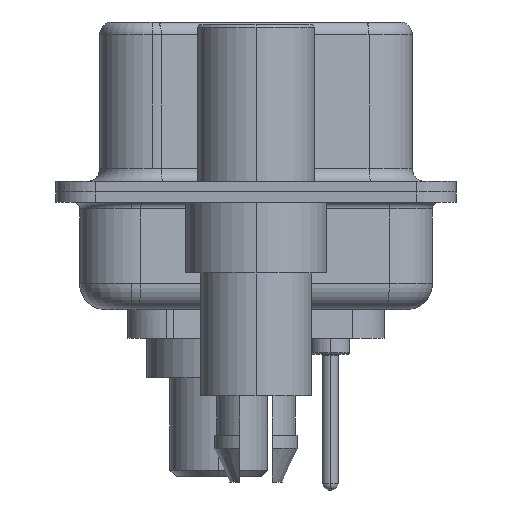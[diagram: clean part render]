
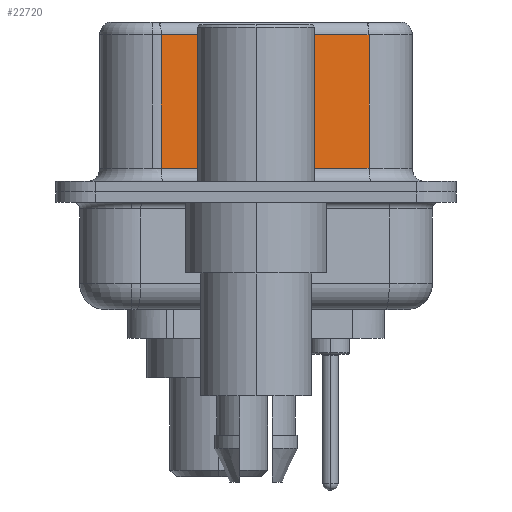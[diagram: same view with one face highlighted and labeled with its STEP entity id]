
A CAD part, left-side view. The second image highlights one B-rep face of the part: STEP entity #22720.
In plain terms, the highlighted planar face has unit normal (-0.985, -0.174, 0).
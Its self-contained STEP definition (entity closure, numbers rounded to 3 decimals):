
#587 = ORIENTED_EDGE ( 'NONE', *, *, #14747, .T. ) ;
#1280 = LINE ( 'NONE', #17066, #16430 ) ;
#2377 = EDGE_CURVE ( 'NONE', #8021, #12807, #23471, .T. ) ;
#3465 = DIRECTION ( 'NONE',  ( -0.174, 0.985, 0. ) ) ;
#3776 = DIRECTION ( 'NONE',  ( -0.174, 0.985, 0. ) ) ;
#4102 = CARTESIAN_POINT ( 'NONE',  ( 5.132, -4.322, 0.9 ) ) ;
#4895 = VERTEX_POINT ( 'NONE', #10823 ) ;
#5987 = DIRECTION ( 'NONE',  ( 0.174, -0.985, 0. ) ) ;
#6564 = ORIENTED_EDGE ( 'NONE', *, *, #2377, .F. ) ;
#7242 = AXIS2_PLACEMENT_3D ( 'NONE', #20576, #14840, #3465 ) ;
#7316 = LINE ( 'NONE', #14742, #21986 ) ;
#8021 = VERTEX_POINT ( 'NONE', #11078 ) ;
#8218 = VECTOR ( 'NONE', #22270, 1000. ) ;
#8408 = CARTESIAN_POINT ( 'NONE',  ( 5.132, -4.322, 6.52 ) ) ;
#8663 = EDGE_LOOP ( 'NONE', ( #6564, #16551, #20786, #587 ) ) ;
#8759 = LINE ( 'NONE', #4102, #18279 ) ;
#9136 = PLANE ( 'NONE',  #7242 ) ;
#9453 = CARTESIAN_POINT ( 'NONE',  ( 3.73, 3.628, 0.9 ) ) ;
#10268 = FACE_OUTER_BOUND ( 'NONE', #8663, .T. ) ;
#10823 = CARTESIAN_POINT ( 'NONE',  ( 3.73, 3.628, 6.02 ) ) ;
#11078 = CARTESIAN_POINT ( 'NONE',  ( 5.132, -4.322, 6.02 ) ) ;
#12807 = VERTEX_POINT ( 'NONE', #22463 ) ;
#12854 = DIRECTION ( 'NONE',  ( 0., 0., -1. ) ) ;
#14634 = EDGE_CURVE ( 'NONE', #8021, #4895, #1280, .T. ) ;
#14742 = CARTESIAN_POINT ( 'NONE',  ( 3.73, 3.628, 6.52 ) ) ;
#14747 = EDGE_CURVE ( 'NONE', #16236, #12807, #8759, .T. ) ;
#14840 = DIRECTION ( 'NONE',  ( 0.985, 0.174, 0. ) ) ;
#16236 = VERTEX_POINT ( 'NONE', #9453 ) ;
#16430 = VECTOR ( 'NONE', #3776, 1000. ) ;
#16551 = ORIENTED_EDGE ( 'NONE', *, *, #14634, .T. ) ;
#17066 = CARTESIAN_POINT ( 'NONE',  ( 5.132, -4.322, 6.02 ) ) ;
#18279 = VECTOR ( 'NONE', #5987, 1000. ) ;
#20576 = CARTESIAN_POINT ( 'NONE',  ( 5.132, -4.322, 6.52 ) ) ;
#20776 = EDGE_CURVE ( 'NONE', #4895, #16236, #7316, .T. ) ;
#20786 = ORIENTED_EDGE ( 'NONE', *, *, #20776, .T. ) ;
#21986 = VECTOR ( 'NONE', #12854, 1000. ) ;
#22270 = DIRECTION ( 'NONE',  ( 0., 0., -1. ) ) ;
#22463 = CARTESIAN_POINT ( 'NONE',  ( 5.132, -4.322, 0.9 ) ) ;
#22720 = ADVANCED_FACE ( 'NONE', ( #10268 ), #9136, .F. ) ;
#23471 = LINE ( 'NONE', #8408, #8218 ) ;
